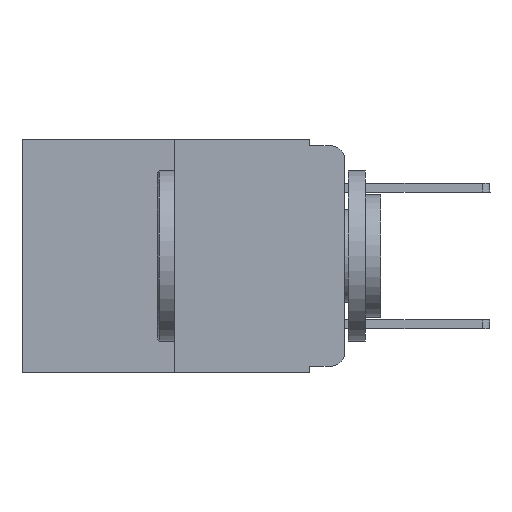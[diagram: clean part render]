
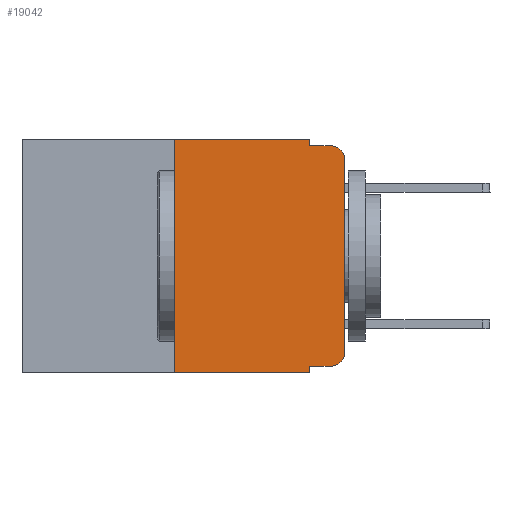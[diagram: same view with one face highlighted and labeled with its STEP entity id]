
A CAD part, left-side view. The second image highlights one B-rep face of the part: STEP entity #19042.
In plain terms, the highlighted planar face has unit normal (-1, 0, 0).
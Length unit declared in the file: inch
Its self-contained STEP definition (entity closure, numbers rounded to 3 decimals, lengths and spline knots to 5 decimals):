
#299 = VECTOR ( 'NONE', #2938, 39.37008 ) ;
#679 = CARTESIAN_POINT ( 'NONE',  ( 0., 0.051, -0.01 ) ) ;
#792 = VERTEX_POINT ( 'NONE', #4400 ) ;
#1166 = LINE ( 'NONE', #5256, #17530 ) ;
#1198 = CARTESIAN_POINT ( 'NONE',  ( 0., 0.051, -0.01 ) ) ;
#1775 = PLANE ( 'NONE',  #18888 ) ;
#1847 = EDGE_CURVE ( 'NONE', #6461, #13867, #24462, .T. ) ;
#2796 = ORIENTED_EDGE ( 'NONE', *, *, #5418, .F. ) ;
#2938 = DIRECTION ( 'NONE',  ( 0., -1., 0. ) ) ;
#3196 = CARTESIAN_POINT ( 'NONE',  ( 0., 0.051, -0.333 ) ) ;
#3593 = AXIS2_PLACEMENT_3D ( 'NONE', #18437, #6487, #6254 ) ;
#3601 = LINE ( 'NONE', #16622, #15128 ) ;
#3700 = EDGE_LOOP ( 'NONE', ( #17431, #11568, #2796, #16234, #5227, #17532, #20744, #11479, #8617, #14275 ) ) ;
#3950 = VERTEX_POINT ( 'NONE', #12851 ) ;
#4400 = CARTESIAN_POINT ( 'NONE',  ( 0., 0., -0.313 ) ) ;
#5227 = ORIENTED_EDGE ( 'NONE', *, *, #1847, .F. ) ;
#5256 = CARTESIAN_POINT ( 'NONE',  ( 0., 0.051, 0. ) ) ;
#5418 = EDGE_CURVE ( 'NONE', #19295, #13982, #17122, .T. ) ;
#5477 = FACE_OUTER_BOUND ( 'NONE', #3700, .T. ) ;
#5938 = DIRECTION ( 'NONE',  ( 0., 0., 1. ) ) ;
#6254 = DIRECTION ( 'NONE',  ( 0., 0., -1. ) ) ;
#6461 = VERTEX_POINT ( 'NONE', #7895 ) ;
#6487 = DIRECTION ( 'NONE',  ( -1., 0., 0. ) ) ;
#6900 = VERTEX_POINT ( 'NONE', #17758 ) ;
#7117 = DIRECTION ( 'NONE',  ( 0., -1., 0. ) ) ;
#7895 = CARTESIAN_POINT ( 'NONE',  ( 0., 0.25, 0. ) ) ;
#8108 = CIRCLE ( 'NONE', #19971, 0.02 ) ;
#8141 = VECTOR ( 'NONE', #12409, 39.37008 ) ;
#8617 = ORIENTED_EDGE ( 'NONE', *, *, #9094, .T. ) ;
#9094 = EDGE_CURVE ( 'NONE', #23647, #3950, #16794, .T. ) ;
#9241 = DIRECTION ( 'NONE',  ( 0., 0., -1. ) ) ;
#9390 = EDGE_CURVE ( 'NONE', #6900, #13982, #17120, .T. ) ;
#9597 = CARTESIAN_POINT ( 'NONE',  ( 0., 0.473, 0. ) ) ;
#10174 = LINE ( 'NONE', #23550, #22986 ) ;
#10354 = VECTOR ( 'NONE', #7117, 39.37008 ) ;
#10851 = CARTESIAN_POINT ( 'NONE',  ( 0., 0.25, 0. ) ) ;
#10955 = EDGE_CURVE ( 'NONE', #14852, #13666, #3601, .T. ) ;
#11378 = DIRECTION ( 'NONE',  ( 0., 0., -1. ) ) ;
#11479 = ORIENTED_EDGE ( 'NONE', *, *, #14094, .F. ) ;
#11568 = ORIENTED_EDGE ( 'NONE', *, *, #9390, .T. ) ;
#12409 = DIRECTION ( 'NONE',  ( 0., 0., 1. ) ) ;
#12763 = CARTESIAN_POINT ( 'NONE',  ( 0., 0.051, -0.343 ) ) ;
#12851 = CARTESIAN_POINT ( 'NONE',  ( 0., 0.02, -0.333 ) ) ;
#13666 = VERTEX_POINT ( 'NONE', #12763 ) ;
#13867 = VERTEX_POINT ( 'NONE', #17397 ) ;
#13982 = VERTEX_POINT ( 'NONE', #24046 ) ;
#14094 = EDGE_CURVE ( 'NONE', #23647, #13666, #1166, .T. ) ;
#14275 = ORIENTED_EDGE ( 'NONE', *, *, #14282, .T. ) ;
#14282 = EDGE_CURVE ( 'NONE', #3950, #792, #8108, .T. ) ;
#14852 = VERTEX_POINT ( 'NONE', #23310 ) ;
#15109 = EDGE_CURVE ( 'NONE', #14852, #6461, #16157, .T. ) ;
#15128 = VECTOR ( 'NONE', #17361, 39.37008 ) ;
#16157 = LINE ( 'NONE', #10851, #8141 ) ;
#16234 = ORIENTED_EDGE ( 'NONE', *, *, #18932, .F. ) ;
#16622 = CARTESIAN_POINT ( 'NONE',  ( 0., 0.473, -0.343 ) ) ;
#16794 = LINE ( 'NONE', #24631, #299 ) ;
#17120 = CIRCLE ( 'NONE', #3593, 0.02 ) ;
#17122 = LINE ( 'NONE', #1198, #18091 ) ;
#17361 = DIRECTION ( 'NONE',  ( 0., -1., 0. ) ) ;
#17397 = CARTESIAN_POINT ( 'NONE',  ( 0., 0.051, 0. ) ) ;
#17431 = ORIENTED_EDGE ( 'NONE', *, *, #18535, .T. ) ;
#17530 = VECTOR ( 'NONE', #9241, 39.37008 ) ;
#17532 = ORIENTED_EDGE ( 'NONE', *, *, #15109, .F. ) ;
#17750 = LINE ( 'NONE', #21702, #24245 ) ;
#17758 = CARTESIAN_POINT ( 'NONE',  ( 0., 0., -0.03 ) ) ;
#18091 = VECTOR ( 'NONE', #18662, 39.37008 ) ;
#18437 = CARTESIAN_POINT ( 'NONE',  ( 0., 0.02, -0.03 ) ) ;
#18535 = EDGE_CURVE ( 'NONE', #792, #6900, #10174, .T. ) ;
#18662 = DIRECTION ( 'NONE',  ( 0., -1., 0. ) ) ;
#18673 = CARTESIAN_POINT ( 'NONE',  ( 0., 0.473, 0. ) ) ;
#18888 = AXIS2_PLACEMENT_3D ( 'NONE', #9597, #25008, #11378 ) ;
#18932 = EDGE_CURVE ( 'NONE', #13867, #19295, #17750, .T. ) ;
#19042 = ADVANCED_FACE ( 'NONE', ( #5477 ), #1775, .F. ) ;
#19295 = VERTEX_POINT ( 'NONE', #679 ) ;
#19527 = CARTESIAN_POINT ( 'NONE',  ( 0., 0.02, -0.313 ) ) ;
#19971 = AXIS2_PLACEMENT_3D ( 'NONE', #19527, #23006, #21070 ) ;
#20744 = ORIENTED_EDGE ( 'NONE', *, *, #10955, .T. ) ;
#21070 = DIRECTION ( 'NONE',  ( 0., 0., -1. ) ) ;
#21702 = CARTESIAN_POINT ( 'NONE',  ( 0., 0.051, 0. ) ) ;
#22986 = VECTOR ( 'NONE', #5938, 39.37008 ) ;
#23006 = DIRECTION ( 'NONE',  ( -1., 0., 0. ) ) ;
#23253 = DIRECTION ( 'NONE',  ( 0., 0., -1. ) ) ;
#23310 = CARTESIAN_POINT ( 'NONE',  ( 0., 0.25, -0.343 ) ) ;
#23550 = CARTESIAN_POINT ( 'NONE',  ( 0., 0., 0. ) ) ;
#23647 = VERTEX_POINT ( 'NONE', #3196 ) ;
#24046 = CARTESIAN_POINT ( 'NONE',  ( 0., 0.02, -0.01 ) ) ;
#24245 = VECTOR ( 'NONE', #23253, 39.37008 ) ;
#24462 = LINE ( 'NONE', #18673, #10354 ) ;
#24631 = CARTESIAN_POINT ( 'NONE',  ( 0., 0.051, -0.333 ) ) ;
#25008 = DIRECTION ( 'NONE',  ( 1., 0., 0. ) ) ;
